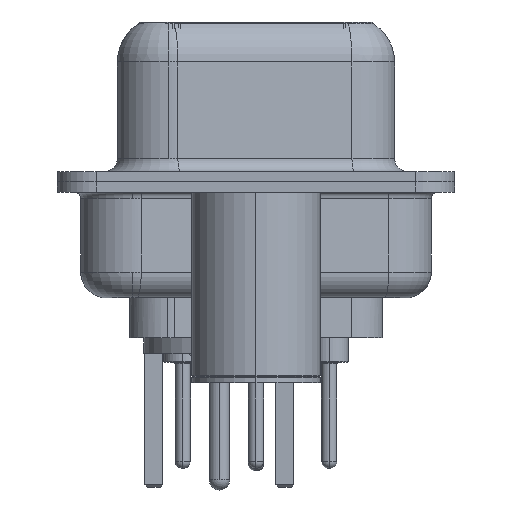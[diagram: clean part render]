
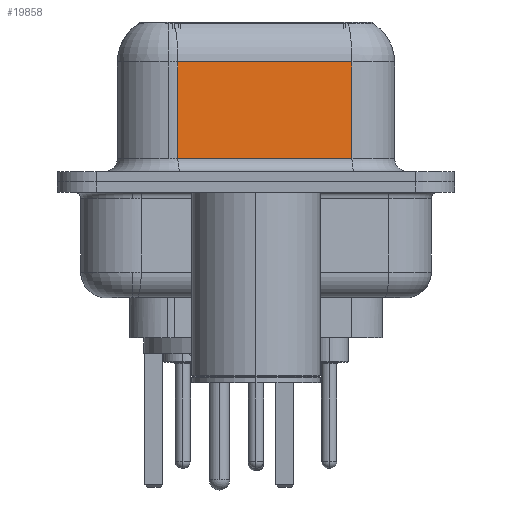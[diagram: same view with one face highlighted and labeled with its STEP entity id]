
A CAD part, left-side view. The second image highlights one B-rep face of the part: STEP entity #19858.
In plain terms, the highlighted planar face has unit normal (-0.985, -0.174, 0).
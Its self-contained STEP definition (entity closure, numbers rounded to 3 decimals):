
#1883 = CARTESIAN_POINT ( 'NONE',  ( 5.621, -3.722, 0.9 ) ) ;
#3330 = VECTOR ( 'NONE', #8949, 1000. ) ;
#3335 = AXIS2_PLACEMENT_3D ( 'NONE', #27905, #30643, #30875 ) ;
#4050 = VERTEX_POINT ( 'NONE', #7251 ) ;
#4883 = ORIENTED_EDGE ( 'NONE', *, *, #9834, .F. ) ;
#5134 = VERTEX_POINT ( 'NONE', #27486 ) ;
#6126 = CARTESIAN_POINT ( 'NONE',  ( 4.43, 3.028, 6.4 ) ) ;
#6464 = PLANE ( 'NONE',  #3335 ) ;
#7251 = CARTESIAN_POINT ( 'NONE',  ( 5.621, -3.722, 4.65 ) ) ;
#7381 = EDGE_LOOP ( 'NONE', ( #4883, #12623, #25010, #10831 ) ) ;
#8949 = DIRECTION ( 'NONE',  ( 0., 0., -1. ) ) ;
#9558 = LINE ( 'NONE', #26715, #30358 ) ;
#9834 = EDGE_CURVE ( 'NONE', #4050, #34432, #9558, .T. ) ;
#10161 = EDGE_CURVE ( 'NONE', #4050, #5134, #14609, .T. ) ;
#10831 = ORIENTED_EDGE ( 'NONE', *, *, #11943, .T. ) ;
#11943 = EDGE_CURVE ( 'NONE', #30084, #34432, #22593, .T. ) ;
#12623 = ORIENTED_EDGE ( 'NONE', *, *, #10161, .T. ) ;
#13397 = DIRECTION ( 'NONE',  ( 0., 0., -1. ) ) ;
#14607 = FACE_OUTER_BOUND ( 'NONE', #7381, .T. ) ;
#14609 = LINE ( 'NONE', #28805, #20578 ) ;
#17361 = EDGE_CURVE ( 'NONE', #5134, #30084, #33410, .T. ) ;
#17528 = DIRECTION ( 'NONE',  ( -0.174, 0.985, 0. ) ) ;
#19858 = ADVANCED_FACE ( 'NONE', ( #14607 ), #6464, .F. ) ;
#20578 = VECTOR ( 'NONE', #17528, 1000. ) ;
#20809 = DIRECTION ( 'NONE',  ( 0.174, -0.985, 0. ) ) ;
#22593 = LINE ( 'NONE', #1883, #33628 ) ;
#25010 = ORIENTED_EDGE ( 'NONE', *, *, #17361, .T. ) ;
#25555 = CARTESIAN_POINT ( 'NONE',  ( 4.43, 3.028, 0.9 ) ) ;
#26715 = CARTESIAN_POINT ( 'NONE',  ( 5.621, -3.722, 6.4 ) ) ;
#27486 = CARTESIAN_POINT ( 'NONE',  ( 4.43, 3.028, 4.65 ) ) ;
#27905 = CARTESIAN_POINT ( 'NONE',  ( 5.621, -3.722, 6.4 ) ) ;
#28805 = CARTESIAN_POINT ( 'NONE',  ( 5.621, -3.722, 4.65 ) ) ;
#30084 = VERTEX_POINT ( 'NONE', #25555 ) ;
#30358 = VECTOR ( 'NONE', #13397, 1000. ) ;
#30643 = DIRECTION ( 'NONE',  ( 0.985, 0.174, 0. ) ) ;
#30875 = DIRECTION ( 'NONE',  ( -0.174, 0.985, 0. ) ) ;
#33410 = LINE ( 'NONE', #6126, #3330 ) ;
#33628 = VECTOR ( 'NONE', #20809, 1000. ) ;
#33947 = CARTESIAN_POINT ( 'NONE',  ( 5.621, -3.722, 0.9 ) ) ;
#34432 = VERTEX_POINT ( 'NONE', #33947 ) ;
